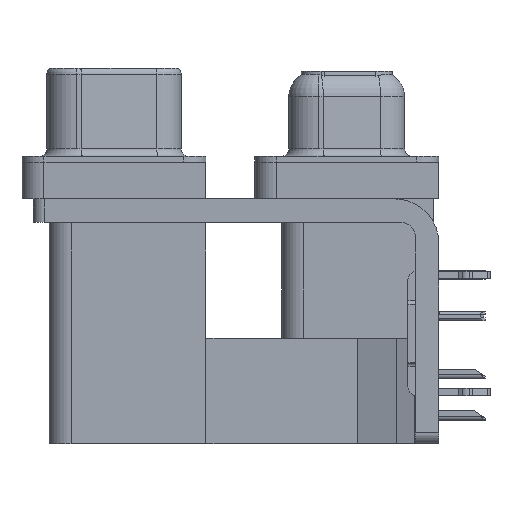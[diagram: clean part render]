
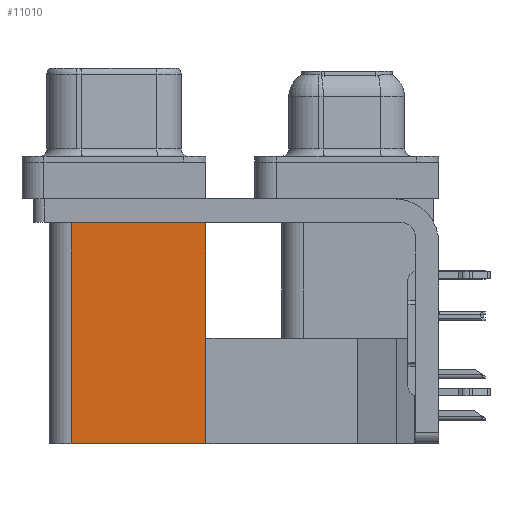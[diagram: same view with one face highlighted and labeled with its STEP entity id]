
A CAD part, left-side view. The second image highlights one B-rep face of the part: STEP entity #11010.
In plain terms, the highlighted planar face has unit normal (-1, 0, 0).
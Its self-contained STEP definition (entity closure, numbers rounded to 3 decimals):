
#822 = CARTESIAN_POINT ( 'NONE',  ( 3.79, 18.8, -2.5 ) ) ;
#1075 = VERTEX_POINT ( 'NONE', #6687 ) ;
#2095 = VERTEX_POINT ( 'NONE', #14903 ) ;
#2306 = LINE ( 'NONE', #39848, #15616 ) ;
#2524 = AXIS2_PLACEMENT_3D ( 'NONE', #39709, #21748, #18721 ) ;
#3661 = DIRECTION ( 'NONE',  ( 0., 1., 0. ) ) ;
#4526 = LINE ( 'NONE', #32410, #32933 ) ;
#5686 = ORIENTED_EDGE ( 'NONE', *, *, #6490, .T. ) ;
#6490 = EDGE_CURVE ( 'NONE', #2095, #38399, #4526, .T. ) ;
#6517 = VECTOR ( 'NONE', #3661, 1000. ) ;
#6687 = CARTESIAN_POINT ( 'NONE',  ( 3.79, 18.8, -19.2 ) ) ;
#7680 = VECTOR ( 'NONE', #24417, 1000. ) ;
#9219 = FACE_OUTER_BOUND ( 'NONE', #24334, .T. ) ;
#9660 = CARTESIAN_POINT ( 'NONE',  ( 3.79, 18.8, -19.2 ) ) ;
#10693 = EDGE_CURVE ( 'NONE', #1075, #38399, #15145, .T. ) ;
#10850 = VERTEX_POINT ( 'NONE', #26610 ) ;
#11010 = ADVANCED_FACE ( 'NONE', ( #9219 ), #12254, .F. ) ;
#12254 = PLANE ( 'NONE',  #2524 ) ;
#14903 = CARTESIAN_POINT ( 'NONE',  ( 3.79, 9.6, -2.5 ) ) ;
#15145 = LINE ( 'NONE', #9660, #7680 ) ;
#15616 = VECTOR ( 'NONE', #31177, 1000. ) ;
#18081 = ORIENTED_EDGE ( 'NONE', *, *, #22542, .F. ) ;
#18721 = DIRECTION ( 'NONE',  ( 0., 0., -1. ) ) ;
#21748 = DIRECTION ( 'NONE',  ( 1., 0., 0. ) ) ;
#22542 = EDGE_CURVE ( 'NONE', #10850, #1075, #28307, .T. ) ;
#24334 = EDGE_LOOP ( 'NONE', ( #5686, #28275, #18081, #32006 ) ) ;
#24417 = DIRECTION ( 'NONE',  ( 0., 0., 1. ) ) ;
#26140 = DIRECTION ( 'NONE',  ( 0., 1., 0. ) ) ;
#26610 = CARTESIAN_POINT ( 'NONE',  ( 3.79, 9.6, -19.2 ) ) ;
#28275 = ORIENTED_EDGE ( 'NONE', *, *, #10693, .F. ) ;
#28307 = LINE ( 'NONE', #31922, #6517 ) ;
#31177 = DIRECTION ( 'NONE',  ( 0., 0., 1. ) ) ;
#31922 = CARTESIAN_POINT ( 'NONE',  ( 3.79, 9.6, -19.2 ) ) ;
#32006 = ORIENTED_EDGE ( 'NONE', *, *, #39476, .T. ) ;
#32410 = CARTESIAN_POINT ( 'NONE',  ( 3.79, 9.6, -2.5 ) ) ;
#32933 = VECTOR ( 'NONE', #26140, 1000. ) ;
#38399 = VERTEX_POINT ( 'NONE', #822 ) ;
#39476 = EDGE_CURVE ( 'NONE', #10850, #2095, #2306, .T. ) ;
#39709 = CARTESIAN_POINT ( 'NONE',  ( 3.79, 9.6, -19.2 ) ) ;
#39848 = CARTESIAN_POINT ( 'NONE',  ( 3.79, 9.6, -19.2 ) ) ;
